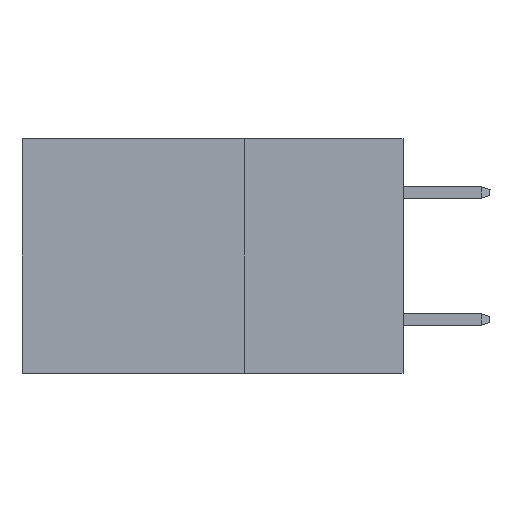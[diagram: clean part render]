
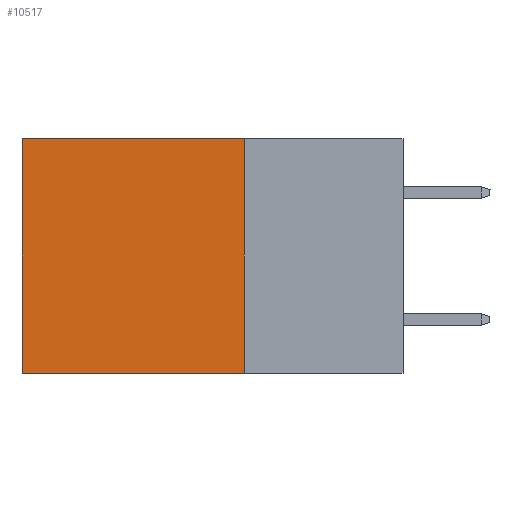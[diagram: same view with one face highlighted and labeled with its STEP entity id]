
A CAD part, left-side view. The second image highlights one B-rep face of the part: STEP entity #10517.
In plain terms, the highlighted planar face has unit normal (-1, 0, 0).
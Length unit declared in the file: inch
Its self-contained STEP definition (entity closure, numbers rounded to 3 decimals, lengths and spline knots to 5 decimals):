
#711 = EDGE_LOOP ( 'NONE', ( #17412, #1899, #11475, #5936 ) ) ;
#1022 = DIRECTION ( 'NONE',  ( 0., 0., -1. ) ) ;
#1899 = ORIENTED_EDGE ( 'NONE', *, *, #17932, .F. ) ;
#2142 = CARTESIAN_POINT ( 'NONE',  ( 0.2875, 0.25, 0. ) ) ;
#2530 = CARTESIAN_POINT ( 'NONE',  ( 0.2875, 0.6, -0.37 ) ) ;
#2695 = CARTESIAN_POINT ( 'NONE',  ( 0.2875, 0.25, 0. ) ) ;
#3594 = VECTOR ( 'NONE', #9523, 39.37008 ) ;
#3932 = EDGE_CURVE ( 'NONE', #17853, #15596, #16954, .T. ) ;
#3980 = PLANE ( 'NONE',  #11721 ) ;
#4523 = LINE ( 'NONE', #2695, #20871 ) ;
#5091 = CARTESIAN_POINT ( 'NONE',  ( 0.2875, 0.25, 0. ) ) ;
#5936 = ORIENTED_EDGE ( 'NONE', *, *, #3932, .T. ) ;
#5985 = LINE ( 'NONE', #7634, #3594 ) ;
#7503 = FACE_OUTER_BOUND ( 'NONE', #711, .T. ) ;
#7634 = CARTESIAN_POINT ( 'NONE',  ( 0.2875, 0.25, -0.37 ) ) ;
#8785 = CARTESIAN_POINT ( 'NONE',  ( 0.2875, 0.6, 0. ) ) ;
#9523 = DIRECTION ( 'NONE',  ( 0., 1., 0. ) ) ;
#9880 = VERTEX_POINT ( 'NONE', #2530 ) ;
#10318 = CARTESIAN_POINT ( 'NONE',  ( 0.2875, 0.25, -0.37 ) ) ;
#10412 = CARTESIAN_POINT ( 'NONE',  ( 0.2875, 0.6, 0. ) ) ;
#10517 = ADVANCED_FACE ( 'NONE', ( #7503 ), #3980, .F. ) ;
#10721 = DIRECTION ( 'NONE',  ( 0., 0., -1. ) ) ;
#11475 = ORIENTED_EDGE ( 'NONE', *, *, #21620, .F. ) ;
#11721 = AXIS2_PLACEMENT_3D ( 'NONE', #17612, #15932, #10721 ) ;
#11793 = VERTEX_POINT ( 'NONE', #10318 ) ;
#13393 = DIRECTION ( 'NONE',  ( 0., 1., 0. ) ) ;
#13735 = LINE ( 'NONE', #10412, #18319 ) ;
#14866 = EDGE_CURVE ( 'NONE', #15596, #9880, #13735, .T. ) ;
#15596 = VERTEX_POINT ( 'NONE', #8785 ) ;
#15932 = DIRECTION ( 'NONE',  ( 1., 0., 0. ) ) ;
#16954 = LINE ( 'NONE', #5091, #18780 ) ;
#17189 = DIRECTION ( 'NONE',  ( 0., 0., -1. ) ) ;
#17412 = ORIENTED_EDGE ( 'NONE', *, *, #14866, .T. ) ;
#17612 = CARTESIAN_POINT ( 'NONE',  ( 0.2875, 0.25, 0. ) ) ;
#17853 = VERTEX_POINT ( 'NONE', #2142 ) ;
#17932 = EDGE_CURVE ( 'NONE', #11793, #9880, #5985, .T. ) ;
#18319 = VECTOR ( 'NONE', #17189, 39.37008 ) ;
#18780 = VECTOR ( 'NONE', #13393, 39.37008 ) ;
#20871 = VECTOR ( 'NONE', #1022, 39.37008 ) ;
#21620 = EDGE_CURVE ( 'NONE', #17853, #11793, #4523, .T. ) ;
